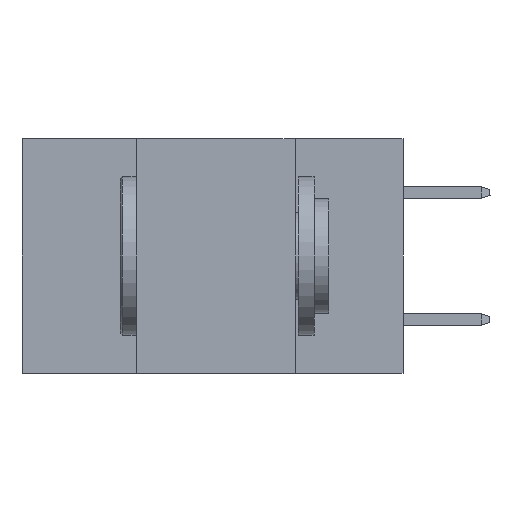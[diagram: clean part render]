
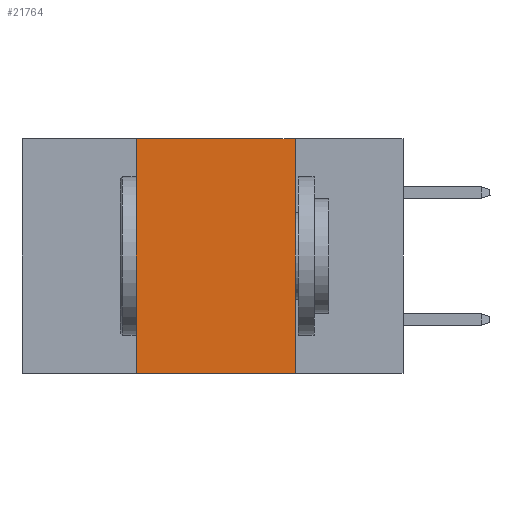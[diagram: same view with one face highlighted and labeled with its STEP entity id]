
A CAD part, left-side view. The second image highlights one B-rep face of the part: STEP entity #21764.
In plain terms, the highlighted planar face has unit normal (-1, 0, 0).
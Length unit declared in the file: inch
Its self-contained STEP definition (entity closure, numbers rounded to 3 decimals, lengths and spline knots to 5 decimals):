
#646 = LINE ( 'NONE', #22099, #28802 ) ;
#1399 = VERTEX_POINT ( 'NONE', #26808 ) ;
#3451 = CARTESIAN_POINT ( 'NONE',  ( 0., 0.17, -0.37 ) ) ;
#5656 = ORIENTED_EDGE ( 'NONE', *, *, #19169, .T. ) ;
#5992 = LINE ( 'NONE', #30134, #22517 ) ;
#8343 = DIRECTION ( 'NONE',  ( 1., 0., 0. ) ) ;
#8617 = DIRECTION ( 'NONE',  ( 0., -1., 0. ) ) ;
#10166 = EDGE_LOOP ( 'NONE', ( #18193, #24324, #17541, #5656 ) ) ;
#11996 = VERTEX_POINT ( 'NONE', #3451 ) ;
#14202 = DIRECTION ( 'NONE',  ( 0., 0., 1. ) ) ;
#14718 = LINE ( 'NONE', #17714, #26781 ) ;
#16536 = VERTEX_POINT ( 'NONE', #32026 ) ;
#17414 = LINE ( 'NONE', #33844, #19572 ) ;
#17541 = ORIENTED_EDGE ( 'NONE', *, *, #33240, .F. ) ;
#17714 = CARTESIAN_POINT ( 'NONE',  ( 0., 0.6, -0.37 ) ) ;
#18193 = ORIENTED_EDGE ( 'NONE', *, *, #26584, .F. ) ;
#19169 = EDGE_CURVE ( 'NONE', #16536, #11996, #14718, .T. ) ;
#19572 = VECTOR ( 'NONE', #30520, 39.37008 ) ;
#21302 = VERTEX_POINT ( 'NONE', #21650 ) ;
#21650 = CARTESIAN_POINT ( 'NONE',  ( 0., 0.17, 0. ) ) ;
#21764 = ADVANCED_FACE ( 'NONE', ( #27390 ), #29842, .F. ) ;
#22099 = CARTESIAN_POINT ( 'NONE',  ( 0., 0.42, 0. ) ) ;
#22517 = VECTOR ( 'NONE', #8617, 39.37008 ) ;
#24324 = ORIENTED_EDGE ( 'NONE', *, *, #31562, .F. ) ;
#26584 = EDGE_CURVE ( 'NONE', #21302, #11996, #17414, .T. ) ;
#26781 = VECTOR ( 'NONE', #30638, 39.37008 ) ;
#26808 = CARTESIAN_POINT ( 'NONE',  ( 0., 0.42, 0. ) ) ;
#27390 = FACE_OUTER_BOUND ( 'NONE', #10166, .T. ) ;
#27498 = AXIS2_PLACEMENT_3D ( 'NONE', #29674, #8343, #32609 ) ;
#28802 = VECTOR ( 'NONE', #14202, 39.37008 ) ;
#29674 = CARTESIAN_POINT ( 'NONE',  ( 0., 0.6, 0. ) ) ;
#29842 = PLANE ( 'NONE',  #27498 ) ;
#30134 = CARTESIAN_POINT ( 'NONE',  ( 0., 0.6, 0. ) ) ;
#30520 = DIRECTION ( 'NONE',  ( 0., 0., -1. ) ) ;
#30638 = DIRECTION ( 'NONE',  ( 0., -1., 0. ) ) ;
#31562 = EDGE_CURVE ( 'NONE', #1399, #21302, #5992, .T. ) ;
#32026 = CARTESIAN_POINT ( 'NONE',  ( 0., 0.42, -0.37 ) ) ;
#32609 = DIRECTION ( 'NONE',  ( 0., 0., -1. ) ) ;
#33240 = EDGE_CURVE ( 'NONE', #16536, #1399, #646, .T. ) ;
#33844 = CARTESIAN_POINT ( 'NONE',  ( 0., 0.17, 0. ) ) ;
